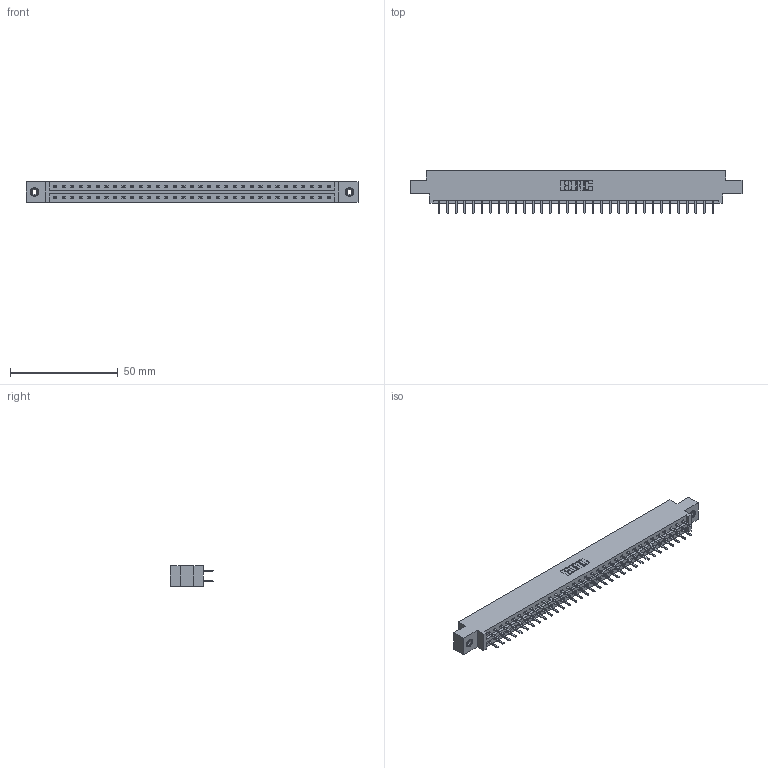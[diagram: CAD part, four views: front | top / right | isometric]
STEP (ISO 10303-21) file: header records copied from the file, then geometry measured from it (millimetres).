
FILE_DESCRIPTION (( 'STEP AP203' ), '1' );
FILE_NAME ('387-066-520-808.STEP', '2018-09-21T09:06:58', ( '' ), ( '' ), 'SwSTEP 2.0', 'SolidWorks 2016', '' );
FILE_SCHEMA (( 'CONFIG_CONTROL_DESIGN' ));
Length unit declared in the file: inch
Products named in the file (4): 337 Part_0.170 Offset - 0.156 Dia-TI; 345-292-001_345-293-120; 345-250-001_345-250-003-102; 387-066-520-808
Assembly tree (69 placements, depth 2):
  387-066-520-808
    337 Part_0.170 Offset - 0.156 Dia-TI
    345-292-001_345-293-120  x66
    345-250-001_345-250-003-102  x2
Bounding box: 153.77 x 20.02 x 9.4 mm (x, y, z)
Volume: 15932.8 mm3; surface area: 17973.7 mm2
Topology: 69 solids, 69 shells, 4006 faces, 11613 edges, 7558 vertices
Faces by surface type: plane 2746, cylinder 1244, cone 12, torus 4
Entity records: 28182 total; most frequent: CARTESIAN_POINT 4749, ORIENTED_EDGE 4666, DIRECTION 4075, EDGE_CURVE 2333, LINE 2181, VECTOR 2181, VERTEX_POINT 1548, AXIS2_PLACEMENT_3D 947
